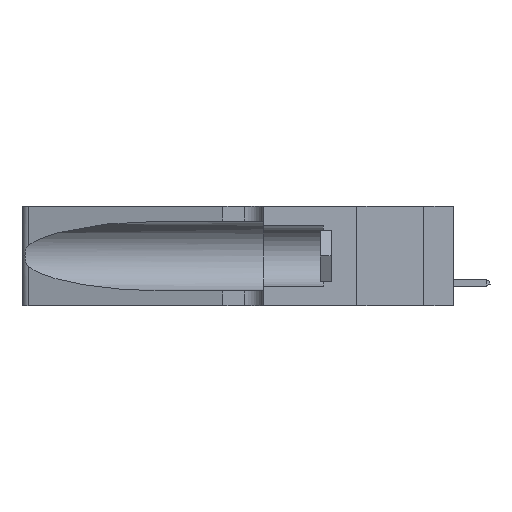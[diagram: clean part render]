
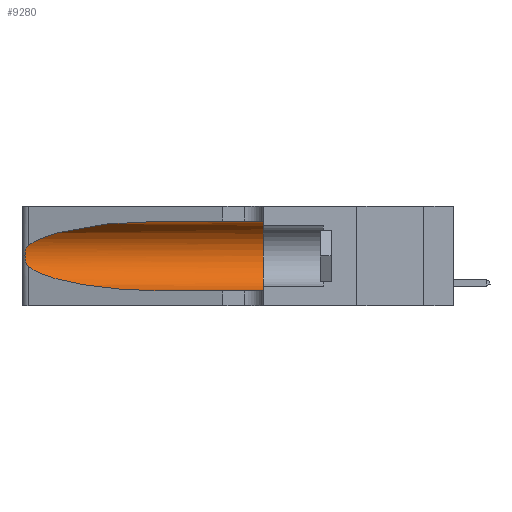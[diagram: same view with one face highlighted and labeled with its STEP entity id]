
A CAD part, left-side view. The second image highlights one B-rep face of the part: STEP entity #9280.
In plain terms, the highlighted cylindrical face has radius 3.308 mm (diameter 6.617 mm), a partial arc.
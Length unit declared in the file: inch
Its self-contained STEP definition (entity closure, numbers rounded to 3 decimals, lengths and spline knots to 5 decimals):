
#257 = FACE_OUTER_BOUND ( 'NONE', #5066, .T. ) ;
#527 = CARTESIAN_POINT ( 'NONE',  ( 0.25787, 1.23484, 0.2124 ) ) ;
#627 = CARTESIAN_POINT ( 'NONE',  ( 0.25487, 1.22718, 0.22369 ) ) ;
#750 = VECTOR ( 'NONE', #14636, 39.37008 ) ;
#1750 = DIRECTION ( 'NONE',  ( 0., -1., 0. ) ) ;
#3651 = CARTESIAN_POINT ( 'NONE',  ( 0.25639, 1.23184, 0.21858 ) ) ;
#3721 = CARTESIAN_POINT ( 'NONE',  ( 0.1305, 1.61858, 0.185 ) ) ;
#3777 = CARTESIAN_POINT ( 'NONE',  ( 0.25789, 1.23486, 0.15765 ) ) ;
#3854 = CARTESIAN_POINT ( 'NONE',  ( 0.1305, 0.35, 0.05475 ) ) ;
#4026 = CARTESIAN_POINT ( 'NONE',  ( 0.1305, 0.72297, 0.31525 ) ) ;
#4211 = VECTOR ( 'NONE', #14085, 39.37008 ) ;
#5066 = EDGE_LOOP ( 'NONE', ( #33420, #23303, #6584, #24271, #29186, #8202 ) ) ;
#6584 = ORIENTED_EDGE ( 'NONE', *, *, #17572, .T. ) ;
#6722 = CARTESIAN_POINT ( 'NONE',  ( 0.26017, 1.23833, 0.17102 ) ) ;
#7008 = CARTESIAN_POINT ( 'NONE',  ( 0.25856, 1.23593, 0.16098 ) ) ;
#7918 = CARTESIAN_POINT ( 'NONE',  ( 0.25487, 1.22718, 0.14631 ) ) ;
#8202 = ORIENTED_EDGE ( 'NONE', *, *, #15809, .F. ) ;
#9280 = ADVANCED_FACE ( 'NONE', ( #257 ), #14215, .F. ) ;
#9314 = CARTESIAN_POINT ( 'NONE',  ( 0.1305, 0.35, 0.185 ) ) ;
#9974 =( BOUNDED_CURVE ( )  B_SPLINE_CURVE ( 3, ( #4026, #10188, #12813, #627 ),
 .UNSPECIFIED., .F., .T. ) 
 B_SPLINE_CURVE_WITH_KNOTS ( ( 4, 4 ),
 ( 1.5708, 2.84003 ),
 .UNSPECIFIED. ) 
 CURVE ( )  GEOMETRIC_REPRESENTATION_ITEM ( )  RATIONAL_B_SPLINE_CURVE ( ( 1., 0.87, 0.87, 1. ) ) 
 REPRESENTATION_ITEM ( '' )  );
#10188 = CARTESIAN_POINT ( 'NONE',  ( 0.18966, 0.96281, 0.31525 ) ) ;
#10505 = VERTEX_POINT ( 'NONE', #39240 ) ;
#10544 = CARTESIAN_POINT ( 'NONE',  ( 0.1305, 0.35, 0.31525 ) ) ;
#12189 = CARTESIAN_POINT ( 'NONE',  ( 0.1305, 0.72297, 0.31525 ) ) ;
#12813 = CARTESIAN_POINT ( 'NONE',  ( 0.2373, 1.15595, 0.28018 ) ) ;
#13566 = VERTEX_POINT ( 'NONE', #10544 ) ;
#13902 = CARTESIAN_POINT ( 'NONE',  ( 0.1305, 0.72297, 0.05475 ) ) ;
#14085 = DIRECTION ( 'NONE',  ( 0., -1., 0. ) ) ;
#14215 = CYLINDRICAL_SURFACE ( 'NONE', #33516, 0.13025 ) ;
#14636 = DIRECTION ( 'NONE',  ( 0., -1., 0. ) ) ;
#15809 = EDGE_CURVE ( 'NONE', #20787, #13566, #24640, .T. ) ;
#15902 = DIRECTION ( 'NONE',  ( 0., 1., 0. ) ) ;
#17572 = EDGE_CURVE ( 'NONE', #31053, #10505, #20022, .T. ) ;
#17676 = VERTEX_POINT ( 'NONE', #3854 ) ;
#17684 = CARTESIAN_POINT ( 'NONE',  ( 0.1305, 1.61858, 0.05475 ) ) ;
#18644 = CIRCLE ( 'NONE', #26796, 0.13025 ) ;
#19127 = CARTESIAN_POINT ( 'NONE',  ( 0.26075, 1.23896, 0.178 ) ) ;
#20022 =( BOUNDED_CURVE ( )  B_SPLINE_CURVE ( 3, ( #7918, #20035, #38124, #13902 ),
 .UNSPECIFIED., .F., .T. ) 
 B_SPLINE_CURVE_WITH_KNOTS ( ( 4, 4 ),
 ( 3.44316, 4.71239 ),
 .UNSPECIFIED. ) 
 CURVE ( )  GEOMETRIC_REPRESENTATION_ITEM ( )  RATIONAL_B_SPLINE_CURVE ( ( 1., 0.87, 0.87, 1. ) ) 
 REPRESENTATION_ITEM ( '' )  );
#20035 = CARTESIAN_POINT ( 'NONE',  ( 0.2373, 1.15595, 0.08982 ) ) ;
#20551 = B_SPLINE_CURVE_WITH_KNOTS ( 'NONE', 3,
 ( #37069, #21910, #3651, #527, #25216, #31332, #24953, #19127, #6722, #7008, #3777, #27736, #28138, #30801 ),
 .UNSPECIFIED., .F., .F.,
 ( 4, 2, 2, 2, 2, 2, 4 ),
 ( 0., 0.00027, 0.00053, 0.00107, 0.0016, 0.00187, 0.00214 ),
 .UNSPECIFIED. ) ;
#20787 = VERTEX_POINT ( 'NONE', #12189 ) ;
#21373 = EDGE_CURVE ( 'NONE', #20787, #38783, #9974, .T. ) ;
#21910 = CARTESIAN_POINT ( 'NONE',  ( 0.25555, 1.22994, 0.2215 ) ) ;
#23303 = ORIENTED_EDGE ( 'NONE', *, *, #32621, .T. ) ;
#24271 = ORIENTED_EDGE ( 'NONE', *, *, #35115, .T. ) ;
#24640 = LINE ( 'NONE', #32819, #750 ) ;
#24953 = CARTESIAN_POINT ( 'NONE',  ( 0.26075, 1.23896, 0.19203 ) ) ;
#25216 = CARTESIAN_POINT ( 'NONE',  ( 0.25854, 1.2359, 0.20912 ) ) ;
#26796 = AXIS2_PLACEMENT_3D ( 'NONE', #9314, #15902, #35369 ) ;
#26877 = CARTESIAN_POINT ( 'NONE',  ( 0.25487, 1.22718, 0.22369 ) ) ;
#27736 = CARTESIAN_POINT ( 'NONE',  ( 0.25639, 1.23186, 0.15144 ) ) ;
#27803 = DIRECTION ( 'NONE',  ( 0., 0., -1. ) ) ;
#28138 = CARTESIAN_POINT ( 'NONE',  ( 0.25555, 1.22993, 0.14849 ) ) ;
#29186 = ORIENTED_EDGE ( 'NONE', *, *, #30706, .F. ) ;
#30706 = EDGE_CURVE ( 'NONE', #13566, #17676, #18644, .T. ) ;
#30801 = CARTESIAN_POINT ( 'NONE',  ( 0.25487, 1.22718, 0.14631 ) ) ;
#31053 = VERTEX_POINT ( 'NONE', #33190 ) ;
#31332 = CARTESIAN_POINT ( 'NONE',  ( 0.26018, 1.23835, 0.19895 ) ) ;
#32621 = EDGE_CURVE ( 'NONE', #38783, #31053, #20551, .T. ) ;
#32819 = CARTESIAN_POINT ( 'NONE',  ( 0.1305, 1.61858, 0.31525 ) ) ;
#33190 = CARTESIAN_POINT ( 'NONE',  ( 0.25487, 1.22718, 0.14631 ) ) ;
#33420 = ORIENTED_EDGE ( 'NONE', *, *, #21373, .T. ) ;
#33516 = AXIS2_PLACEMENT_3D ( 'NONE', #3721, #1750, #27803 ) ;
#35115 = EDGE_CURVE ( 'NONE', #10505, #17676, #36161, .T. ) ;
#35369 = DIRECTION ( 'NONE',  ( 0., 0., 1. ) ) ;
#36161 = LINE ( 'NONE', #17684, #4211 ) ;
#37069 = CARTESIAN_POINT ( 'NONE',  ( 0.25487, 1.22718, 0.22369 ) ) ;
#38124 = CARTESIAN_POINT ( 'NONE',  ( 0.18966, 0.96281, 0.05475 ) ) ;
#38783 = VERTEX_POINT ( 'NONE', #26877 ) ;
#39240 = CARTESIAN_POINT ( 'NONE',  ( 0.1305, 0.72297, 0.05475 ) ) ;
